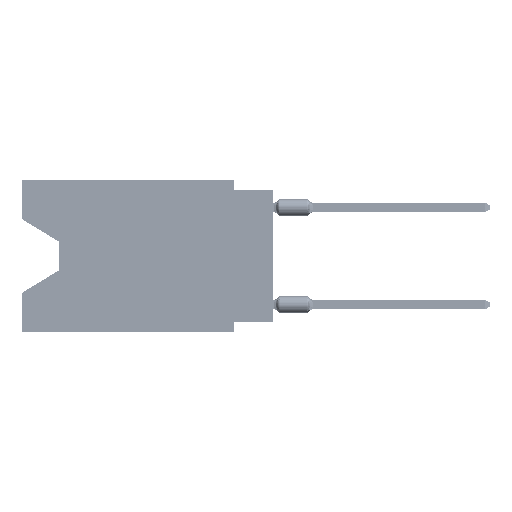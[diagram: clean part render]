
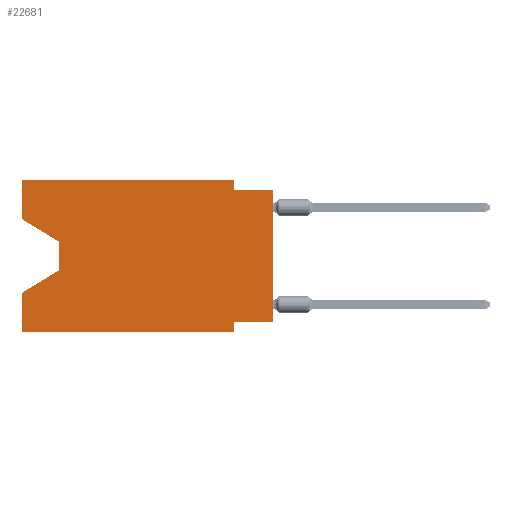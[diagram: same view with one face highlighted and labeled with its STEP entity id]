
A CAD part, left-side view. The second image highlights one B-rep face of the part: STEP entity #22681.
In plain terms, the highlighted planar face has unit normal (-1, 0, 0).
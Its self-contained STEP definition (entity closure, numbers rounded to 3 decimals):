
#362 = VECTOR ( 'NONE', #2664, 1000. ) ;
#988 = ORIENTED_EDGE ( 'NONE', *, *, #35969, .F. ) ;
#2664 = DIRECTION ( 'NONE',  ( 0., -1., 0. ) ) ;
#2777 = DIRECTION ( 'NONE',  ( 0., 0.855, -0.519 ) ) ;
#3561 = VECTOR ( 'NONE', #71394, 1000. ) ;
#3663 = LINE ( 'NONE', #29263, #19074 ) ;
#6933 = VERTEX_POINT ( 'NONE', #34184 ) ;
#7004 = CARTESIAN_POINT ( 'NONE',  ( 0., 13.97, -4.013 ) ) ;
#8163 = CARTESIAN_POINT ( 'NONE',  ( 0., 16.383, 0. ) ) ;
#9110 = CARTESIAN_POINT ( 'NONE',  ( 0., 0., 0. ) ) ;
#9752 = CARTESIAN_POINT ( 'NONE',  ( 0., 2.54, 0. ) ) ;
#10010 = EDGE_CURVE ( 'NONE', #52695, #39096, #58695, .T. ) ;
#10972 = LINE ( 'NONE', #87205, #78935 ) ;
#11509 = EDGE_CURVE ( 'NONE', #59977, #79273, #79055, .T. ) ;
#11525 = DIRECTION ( 'NONE',  ( 0., 0., -1. ) ) ;
#12268 = CARTESIAN_POINT ( 'NONE',  ( 0., 16.383, 0. ) ) ;
#12307 = VECTOR ( 'NONE', #57297, 1000. ) ;
#12546 = VERTEX_POINT ( 'NONE', #21364 ) ;
#12639 = VERTEX_POINT ( 'NONE', #34396 ) ;
#13892 = ORIENTED_EDGE ( 'NONE', *, *, #20413, .F. ) ;
#14784 = ORIENTED_EDGE ( 'NONE', *, *, #10010, .F. ) ;
#15049 = LINE ( 'NONE', #83687, #48255 ) ;
#18526 = ORIENTED_EDGE ( 'NONE', *, *, #20679, .T. ) ;
#19074 = VECTOR ( 'NONE', #2777, 1000. ) ;
#19177 = VECTOR ( 'NONE', #58429, 1000. ) ;
#19732 = ORIENTED_EDGE ( 'NONE', *, *, #48331, .T. ) ;
#20413 = EDGE_CURVE ( 'NONE', #28160, #12546, #10972, .T. ) ;
#20679 = EDGE_CURVE ( 'NONE', #6933, #39096, #36928, .T. ) ;
#21364 = CARTESIAN_POINT ( 'NONE',  ( 0., 16.383, -7.36 ) ) ;
#22681 = ADVANCED_FACE ( 'NONE', ( #62305 ), #26448, .F. ) ;
#22723 = ORIENTED_EDGE ( 'NONE', *, *, #69545, .T. ) ;
#22739 = DIRECTION ( 'NONE',  ( 0., 0., 1. ) ) ;
#24523 = VECTOR ( 'NONE', #41419, 1000. ) ;
#25721 = LINE ( 'NONE', #12268, #24523 ) ;
#26448 = PLANE ( 'NONE',  #61971 ) ;
#28160 = VERTEX_POINT ( 'NONE', #87194 ) ;
#28226 = EDGE_CURVE ( 'NONE', #60583, #37082, #59395, .T. ) ;
#29263 = CARTESIAN_POINT ( 'NONE',  ( 0., 13.97, -5.893 ) ) ;
#31029 = CARTESIAN_POINT ( 'NONE',  ( 0., 0., -9.271 ) ) ;
#31728 = CARTESIAN_POINT ( 'NONE',  ( 0., 13.97, -4.013 ) ) ;
#33883 = ORIENTED_EDGE ( 'NONE', *, *, #61108, .T. ) ;
#34184 = CARTESIAN_POINT ( 'NONE',  ( 0., 0., -9.271 ) ) ;
#34396 = CARTESIAN_POINT ( 'NONE',  ( 0., 13.97, -5.893 ) ) ;
#35969 = EDGE_CURVE ( 'NONE', #6933, #59977, #57948, .T. ) ;
#36503 = CARTESIAN_POINT ( 'NONE',  ( 0., 2.54, -9.906 ) ) ;
#36928 = LINE ( 'NONE', #9110, #60369 ) ;
#37082 = VERTEX_POINT ( 'NONE', #7004 ) ;
#38102 = CARTESIAN_POINT ( 'NONE',  ( 0., 0., -0.635 ) ) ;
#38351 = DIRECTION ( 'NONE',  ( 0., 0., 1. ) ) ;
#38761 = CARTESIAN_POINT ( 'NONE',  ( 0., 2.54, 0. ) ) ;
#39096 = VERTEX_POINT ( 'NONE', #38102 ) ;
#41419 = DIRECTION ( 'NONE',  ( 0., -1., 0. ) ) ;
#42875 = DIRECTION ( 'NONE',  ( 0., -1., 0. ) ) ;
#42956 = CARTESIAN_POINT ( 'NONE',  ( 0., 16.383, 0. ) ) ;
#47235 = VERTEX_POINT ( 'NONE', #38761 ) ;
#47618 = CARTESIAN_POINT ( 'NONE',  ( 0., 2.54, -0.635 ) ) ;
#47897 = EDGE_CURVE ( 'NONE', #47235, #52695, #77936, .T. ) ;
#48255 = VECTOR ( 'NONE', #42875, 1000. ) ;
#48331 = EDGE_CURVE ( 'NONE', #28160, #79273, #15049, .T. ) ;
#48361 = CARTESIAN_POINT ( 'NONE',  ( 0., 2.54, -9.906 ) ) ;
#49928 = DIRECTION ( 'NONE',  ( 0., 0., 1. ) ) ;
#51167 = ORIENTED_EDGE ( 'NONE', *, *, #47897, .F. ) ;
#52695 = VERTEX_POINT ( 'NONE', #47618 ) ;
#53212 = DIRECTION ( 'NONE',  ( 0., 0., -1. ) ) ;
#53806 = CARTESIAN_POINT ( 'NONE',  ( 0., 16.383, 0. ) ) ;
#57297 = DIRECTION ( 'NONE',  ( 0., 0., -1. ) ) ;
#57948 = LINE ( 'NONE', #31029, #3561 ) ;
#58429 = DIRECTION ( 'NONE',  ( 0., 0., -1. ) ) ;
#58644 = LINE ( 'NONE', #31728, #76864 ) ;
#58695 = LINE ( 'NONE', #64554, #362 ) ;
#59395 = LINE ( 'NONE', #86756, #84138 ) ;
#59977 = VERTEX_POINT ( 'NONE', #68530 ) ;
#60369 = VECTOR ( 'NONE', #49928, 1000. ) ;
#60378 = DIRECTION ( 'NONE',  ( 1., 0., 0. ) ) ;
#60583 = VERTEX_POINT ( 'NONE', #83203 ) ;
#61108 = EDGE_CURVE ( 'NONE', #12639, #12546, #3663, .T. ) ;
#61682 = ORIENTED_EDGE ( 'NONE', *, *, #11509, .F. ) ;
#61971 = AXIS2_PLACEMENT_3D ( 'NONE', #53806, #60378, #53212 ) ;
#62305 = FACE_OUTER_BOUND ( 'NONE', #79211, .T. ) ;
#64554 = CARTESIAN_POINT ( 'NONE',  ( 0., 0., -0.635 ) ) ;
#65250 = DIRECTION ( 'NONE',  ( 0., -0.855, -0.519 ) ) ;
#66268 = VECTOR ( 'NONE', #22739, 1000. ) ;
#68530 = CARTESIAN_POINT ( 'NONE',  ( 0., 2.54, -9.271 ) ) ;
#69310 = ORIENTED_EDGE ( 'NONE', *, *, #28226, .T. ) ;
#69545 = EDGE_CURVE ( 'NONE', #37082, #12639, #58644, .T. ) ;
#71359 = VERTEX_POINT ( 'NONE', #8163 ) ;
#71394 = DIRECTION ( 'NONE',  ( 0., 1., 0. ) ) ;
#75873 = ORIENTED_EDGE ( 'NONE', *, *, #86767, .F. ) ;
#76864 = VECTOR ( 'NONE', #11525, 1000. ) ;
#77030 = LINE ( 'NONE', #42956, #66268 ) ;
#77936 = LINE ( 'NONE', #9752, #12307 ) ;
#78935 = VECTOR ( 'NONE', #38351, 1000. ) ;
#79055 = LINE ( 'NONE', #36503, #19177 ) ;
#79211 = EDGE_LOOP ( 'NONE', ( #69310, #22723, #33883, #13892, #19732, #61682, #988, #18526, #14784, #51167, #79973, #75873 ) ) ;
#79273 = VERTEX_POINT ( 'NONE', #48361 ) ;
#79973 = ORIENTED_EDGE ( 'NONE', *, *, #85122, .F. ) ;
#83203 = CARTESIAN_POINT ( 'NONE',  ( 0., 16.383, -2.546 ) ) ;
#83687 = CARTESIAN_POINT ( 'NONE',  ( 0., 16.383, -9.906 ) ) ;
#84138 = VECTOR ( 'NONE', #65250, 1000. ) ;
#85122 = EDGE_CURVE ( 'NONE', #71359, #47235, #25721, .T. ) ;
#86756 = CARTESIAN_POINT ( 'NONE',  ( 0., 16.383, -2.546 ) ) ;
#86767 = EDGE_CURVE ( 'NONE', #60583, #71359, #77030, .T. ) ;
#87194 = CARTESIAN_POINT ( 'NONE',  ( 0., 16.383, -9.906 ) ) ;
#87205 = CARTESIAN_POINT ( 'NONE',  ( 0., 16.383, 0. ) ) ;
